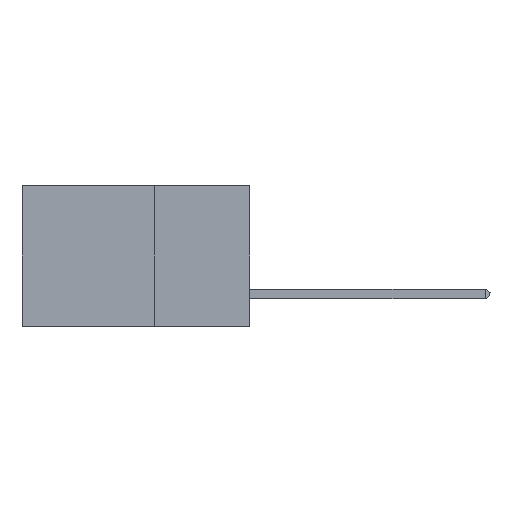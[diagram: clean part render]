
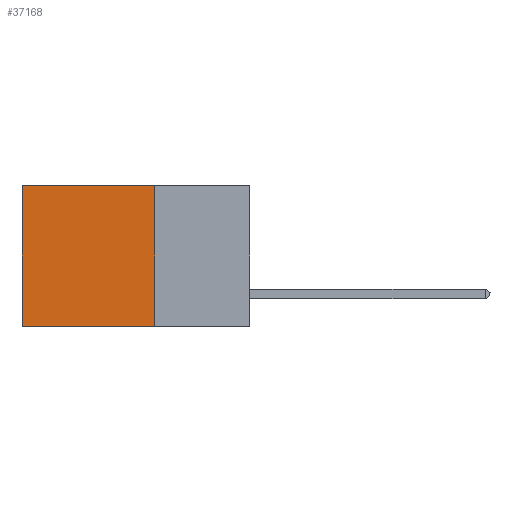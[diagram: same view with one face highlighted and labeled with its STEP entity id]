
A CAD part, left-side view. The second image highlights one B-rep face of the part: STEP entity #37168.
In plain terms, the highlighted planar face has unit normal (-1, 0, 0).
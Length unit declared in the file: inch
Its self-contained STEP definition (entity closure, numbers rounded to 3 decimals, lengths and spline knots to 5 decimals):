
#1353 = VERTEX_POINT ( 'NONE', #47257 ) ;
#1903 = PLANE ( 'NONE',  #30040 ) ;
#5164 = CARTESIAN_POINT ( 'NONE',  ( 0.2875, 0.6, -0.37 ) ) ;
#6255 = VECTOR ( 'NONE', #39877, 39.37008 ) ;
#6771 = ORIENTED_EDGE ( 'NONE', *, *, #22518, .F. ) ;
#7483 = CARTESIAN_POINT ( 'NONE',  ( 0.2875, 0.25, -0.37 ) ) ;
#7837 = DIRECTION ( 'NONE',  ( 0., 0., -1. ) ) ;
#9551 = CARTESIAN_POINT ( 'NONE',  ( 0.2875, 0.25, 0. ) ) ;
#10330 = DIRECTION ( 'NONE',  ( 0., 1., 0. ) ) ;
#13107 = VECTOR ( 'NONE', #40001, 39.37008 ) ;
#13510 = VECTOR ( 'NONE', #7837, 39.37008 ) ;
#14383 = LINE ( 'NONE', #17145, #13107 ) ;
#17145 = CARTESIAN_POINT ( 'NONE',  ( 0.2875, 0.25, -0.37 ) ) ;
#20044 = EDGE_LOOP ( 'NONE', ( #46558, #29563, #6771, #40069 ) ) ;
#20635 = DIRECTION ( 'NONE',  ( 0., 0., -1. ) ) ;
#22518 = EDGE_CURVE ( 'NONE', #1353, #48859, #22838, .T. ) ;
#22838 = LINE ( 'NONE', #35868, #6255 ) ;
#23528 = LINE ( 'NONE', #26696, #13510 ) ;
#24778 = DIRECTION ( 'NONE',  ( 1., 0., 0. ) ) ;
#24917 = EDGE_CURVE ( 'NONE', #48859, #44188, #14383, .T. ) ;
#26696 = CARTESIAN_POINT ( 'NONE',  ( 0.2875, 0.6, 0. ) ) ;
#27037 = EDGE_CURVE ( 'NONE', #47883, #44188, #23528, .T. ) ;
#27384 = VECTOR ( 'NONE', #10330, 39.37008 ) ;
#28619 = CARTESIAN_POINT ( 'NONE',  ( 0.2875, 0.6, 0. ) ) ;
#29166 = CARTESIAN_POINT ( 'NONE',  ( 0.2875, 0.25, 0. ) ) ;
#29563 = ORIENTED_EDGE ( 'NONE', *, *, #24917, .F. ) ;
#30040 = AXIS2_PLACEMENT_3D ( 'NONE', #9551, #24778, #20635 ) ;
#30478 = FACE_OUTER_BOUND ( 'NONE', #20044, .T. ) ;
#33973 = LINE ( 'NONE', #29166, #27384 ) ;
#35868 = CARTESIAN_POINT ( 'NONE',  ( 0.2875, 0.25, 0. ) ) ;
#37168 = ADVANCED_FACE ( 'NONE', ( #30478 ), #1903, .F. ) ;
#37743 = EDGE_CURVE ( 'NONE', #1353, #47883, #33973, .T. ) ;
#39877 = DIRECTION ( 'NONE',  ( 0., 0., -1. ) ) ;
#40001 = DIRECTION ( 'NONE',  ( 0., 1., 0. ) ) ;
#40069 = ORIENTED_EDGE ( 'NONE', *, *, #37743, .T. ) ;
#44188 = VERTEX_POINT ( 'NONE', #5164 ) ;
#46558 = ORIENTED_EDGE ( 'NONE', *, *, #27037, .T. ) ;
#47257 = CARTESIAN_POINT ( 'NONE',  ( 0.2875, 0.25, 0. ) ) ;
#47883 = VERTEX_POINT ( 'NONE', #28619 ) ;
#48859 = VERTEX_POINT ( 'NONE', #7483 ) ;
